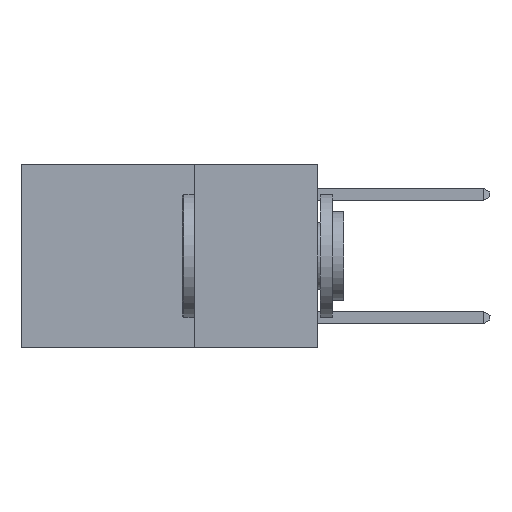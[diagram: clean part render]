
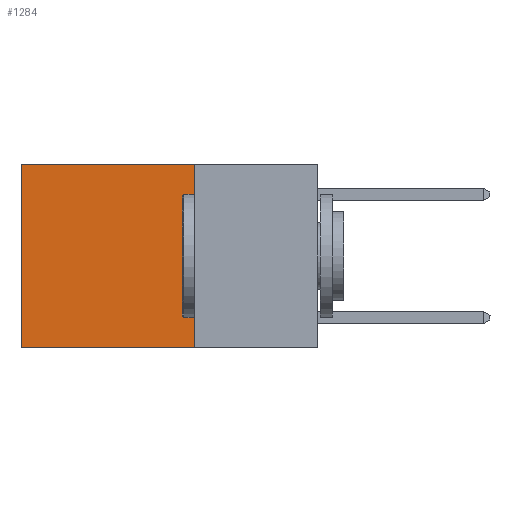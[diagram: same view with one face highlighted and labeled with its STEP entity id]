
A CAD part, left-side view. The second image highlights one B-rep face of the part: STEP entity #1284.
In plain terms, the highlighted planar face has unit normal (-1, 0, 0).
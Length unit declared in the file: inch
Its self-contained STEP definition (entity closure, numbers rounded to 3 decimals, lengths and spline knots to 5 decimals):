
#140 = ORIENTED_EDGE ( 'NONE', *, *, #16873, .T. ) ;
#582 = LINE ( 'NONE', #13822, #12480 ) ;
#777 = VERTEX_POINT ( 'NONE', #11755 ) ;
#898 = LINE ( 'NONE', #3169, #14158 ) ;
#1284 = ADVANCED_FACE ( 'NONE', ( #19320 ), #5786, .F. ) ;
#3169 = CARTESIAN_POINT ( 'NONE',  ( 0.2625, 0.25, -0.37 ) ) ;
#3425 = VERTEX_POINT ( 'NONE', #20539 ) ;
#4510 = EDGE_LOOP ( 'NONE', ( #21799, #18788, #12588, #140 ) ) ;
#5786 = PLANE ( 'NONE',  #14719 ) ;
#5972 = VERTEX_POINT ( 'NONE', #9223 ) ;
#6858 = CARTESIAN_POINT ( 'NONE',  ( 0.2625, 0.6, 0. ) ) ;
#9223 = CARTESIAN_POINT ( 'NONE',  ( 0.2625, 0.25, 0. ) ) ;
#9341 = DIRECTION ( 'NONE',  ( 0., 0., -1. ) ) ;
#9377 = VECTOR ( 'NONE', #21127, 39.37008 ) ;
#11755 = CARTESIAN_POINT ( 'NONE',  ( 0.2625, 0.25, -0.37 ) ) ;
#11946 = LINE ( 'NONE', #22539, #20266 ) ;
#11967 = DIRECTION ( 'NONE',  ( 0., 1., 0. ) ) ;
#12057 = DIRECTION ( 'NONE',  ( 0., 1., 0. ) ) ;
#12480 = VECTOR ( 'NONE', #11967, 39.37008 ) ;
#12521 = EDGE_CURVE ( 'NONE', #3425, #21496, #14070, .T. ) ;
#12588 = ORIENTED_EDGE ( 'NONE', *, *, #16305, .F. ) ;
#12740 = CARTESIAN_POINT ( 'NONE',  ( 0.2625, 0.25, 0. ) ) ;
#13822 = CARTESIAN_POINT ( 'NONE',  ( 0.2625, 0.25, 0. ) ) ;
#14070 = LINE ( 'NONE', #6858, #9377 ) ;
#14158 = VECTOR ( 'NONE', #12057, 39.37008 ) ;
#14719 = AXIS2_PLACEMENT_3D ( 'NONE', #12740, #19870, #9341 ) ;
#15990 = EDGE_CURVE ( 'NONE', #777, #21496, #898, .T. ) ;
#16305 = EDGE_CURVE ( 'NONE', #5972, #777, #11946, .T. ) ;
#16873 = EDGE_CURVE ( 'NONE', #5972, #3425, #582, .T. ) ;
#17224 = DIRECTION ( 'NONE',  ( 0., 0., -1. ) ) ;
#18788 = ORIENTED_EDGE ( 'NONE', *, *, #15990, .F. ) ;
#19320 = FACE_OUTER_BOUND ( 'NONE', #4510, .T. ) ;
#19870 = DIRECTION ( 'NONE',  ( 1., 0., 0. ) ) ;
#19943 = CARTESIAN_POINT ( 'NONE',  ( 0.2625, 0.6, -0.37 ) ) ;
#20266 = VECTOR ( 'NONE', #17224, 39.37008 ) ;
#20539 = CARTESIAN_POINT ( 'NONE',  ( 0.2625, 0.6, 0. ) ) ;
#21127 = DIRECTION ( 'NONE',  ( 0., 0., -1. ) ) ;
#21496 = VERTEX_POINT ( 'NONE', #19943 ) ;
#21799 = ORIENTED_EDGE ( 'NONE', *, *, #12521, .T. ) ;
#22539 = CARTESIAN_POINT ( 'NONE',  ( 0.2625, 0.25, 0. ) ) ;
